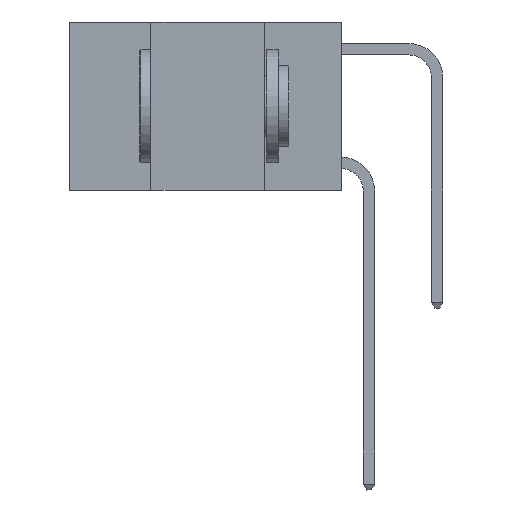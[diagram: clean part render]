
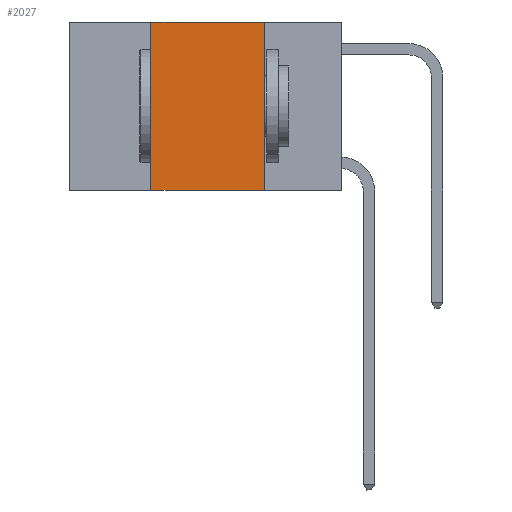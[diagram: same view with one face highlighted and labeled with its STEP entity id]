
A CAD part, left-side view. The second image highlights one B-rep face of the part: STEP entity #2027.
In plain terms, the highlighted planar face has unit normal (-1, 0, 0).
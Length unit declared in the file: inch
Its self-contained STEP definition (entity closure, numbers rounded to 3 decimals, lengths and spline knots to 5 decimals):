
#185 = EDGE_CURVE ( 'NONE', #9566, #1387, #16720, .T. ) ;
#188 = DIRECTION ( 'NONE',  ( 0., 0., 1. ) ) ;
#250 = PLANE ( 'NONE',  #19700 ) ;
#260 = LINE ( 'NONE', #22220, #14844 ) ;
#382 = VERTEX_POINT ( 'NONE', #13952 ) ;
#392 = VECTOR ( 'NONE', #22671, 39.37008 ) ;
#1387 = VERTEX_POINT ( 'NONE', #14343 ) ;
#1867 = CARTESIAN_POINT ( 'NONE',  ( 0., 0.17, -0.37 ) ) ;
#2027 = ADVANCED_FACE ( 'NONE', ( #18725 ), #250, .F. ) ;
#3617 = ORIENTED_EDGE ( 'NONE', *, *, #11601, .T. ) ;
#5999 = EDGE_CURVE ( 'NONE', #382, #9566, #11110, .T. ) ;
#6323 = VECTOR ( 'NONE', #188, 39.37008 ) ;
#9519 = CARTESIAN_POINT ( 'NONE',  ( 0., 0.6, 0. ) ) ;
#9566 = VERTEX_POINT ( 'NONE', #14086 ) ;
#9621 = DIRECTION ( 'NONE',  ( 1., 0., 0. ) ) ;
#11110 = LINE ( 'NONE', #22386, #6323 ) ;
#11119 = VERTEX_POINT ( 'NONE', #1867 ) ;
#11190 = DIRECTION ( 'NONE',  ( 0., -1., 0. ) ) ;
#11601 = EDGE_CURVE ( 'NONE', #382, #11119, #260, .T. ) ;
#13114 = DIRECTION ( 'NONE',  ( 0., 0., -1. ) ) ;
#13952 = CARTESIAN_POINT ( 'NONE',  ( 0., 0.42, -0.37 ) ) ;
#14086 = CARTESIAN_POINT ( 'NONE',  ( 0., 0.42, 0. ) ) ;
#14123 = ORIENTED_EDGE ( 'NONE', *, *, #18398, .F. ) ;
#14343 = CARTESIAN_POINT ( 'NONE',  ( 0., 0.17, 0. ) ) ;
#14844 = VECTOR ( 'NONE', #22102, 39.37008 ) ;
#15357 = CARTESIAN_POINT ( 'NONE',  ( 0., 0.17, 0. ) ) ;
#16330 = VECTOR ( 'NONE', #11190, 39.37008 ) ;
#16720 = LINE ( 'NONE', #9519, #16330 ) ;
#17163 = LINE ( 'NONE', #15357, #392 ) ;
#17780 = EDGE_LOOP ( 'NONE', ( #14123, #22474, #23485, #3617 ) ) ;
#18398 = EDGE_CURVE ( 'NONE', #1387, #11119, #17163, .T. ) ;
#18725 = FACE_OUTER_BOUND ( 'NONE', #17780, .T. ) ;
#19700 = AXIS2_PLACEMENT_3D ( 'NONE', #22560, #9621, #13114 ) ;
#22102 = DIRECTION ( 'NONE',  ( 0., -1., 0. ) ) ;
#22220 = CARTESIAN_POINT ( 'NONE',  ( 0., 0.6, -0.37 ) ) ;
#22386 = CARTESIAN_POINT ( 'NONE',  ( 0., 0.42, 0. ) ) ;
#22474 = ORIENTED_EDGE ( 'NONE', *, *, #185, .F. ) ;
#22560 = CARTESIAN_POINT ( 'NONE',  ( 0., 0.6, 0. ) ) ;
#22671 = DIRECTION ( 'NONE',  ( 0., 0., -1. ) ) ;
#23485 = ORIENTED_EDGE ( 'NONE', *, *, #5999, .F. ) ;
